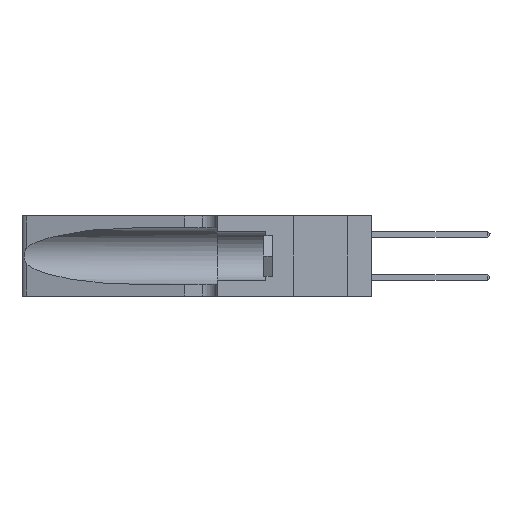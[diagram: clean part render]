
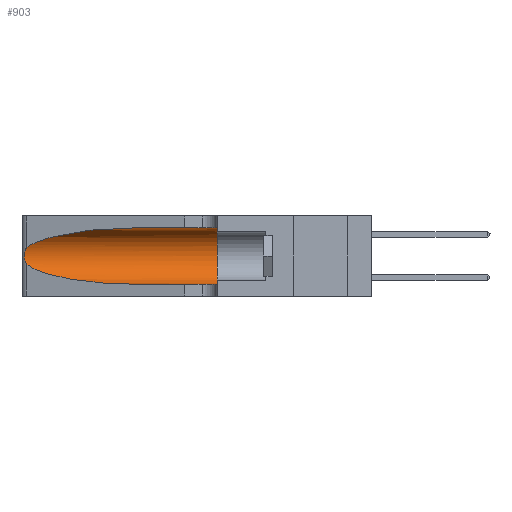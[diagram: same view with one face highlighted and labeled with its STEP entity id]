
A CAD part, left-side view. The second image highlights one B-rep face of the part: STEP entity #903.
In plain terms, the highlighted cylindrical face has radius 3.308 mm (diameter 6.617 mm), a partial arc.
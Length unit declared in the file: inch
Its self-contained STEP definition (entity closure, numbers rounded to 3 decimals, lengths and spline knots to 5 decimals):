
#76 = CARTESIAN_POINT ( 'NONE',  ( 0.1305, 0.72297, 0.05475 ) ) ;
#342 = DIRECTION ( 'NONE',  ( 0., 0., -1. ) ) ;
#652 = DIRECTION ( 'NONE',  ( 0., -1., 0. ) ) ;
#903 = ADVANCED_FACE ( 'NONE', ( #17242 ), #10014, .F. ) ;
#1303 = CARTESIAN_POINT ( 'NONE',  ( 0.25487, 1.22718, 0.22369 ) ) ;
#1406 = CARTESIAN_POINT ( 'NONE',  ( 0.26075, 1.23896, 0.19203 ) ) ;
#1470 = ORIENTED_EDGE ( 'NONE', *, *, #22122, .F. ) ;
#1732 = CARTESIAN_POINT ( 'NONE',  ( 0.1305, 0.72297, 0.31525 ) ) ;
#2048 = DIRECTION ( 'NONE',  ( 0., 1., 0. ) ) ;
#2212 = ORIENTED_EDGE ( 'NONE', *, *, #2371, .T. ) ;
#2371 = EDGE_CURVE ( 'NONE', #25575, #6496, #21791, .T. ) ;
#3704 = CARTESIAN_POINT ( 'NONE',  ( 0.26017, 1.23833, 0.17102 ) ) ;
#5071 = VECTOR ( 'NONE', #652, 39.37008 ) ;
#5984 = CARTESIAN_POINT ( 'NONE',  ( 0.25789, 1.23486, 0.15765 ) ) ;
#6429 = VERTEX_POINT ( 'NONE', #19236 ) ;
#6496 = VERTEX_POINT ( 'NONE', #10642 ) ;
#6513 = ORIENTED_EDGE ( 'NONE', *, *, #19465, .F. ) ;
#6844 = CARTESIAN_POINT ( 'NONE',  ( 0.18966, 0.96281, 0.05475 ) ) ;
#7109 = ORIENTED_EDGE ( 'NONE', *, *, #22461, .T. ) ;
#7920 = CARTESIAN_POINT ( 'NONE',  ( 0.2373, 1.15595, 0.28018 ) ) ;
#8261 = CARTESIAN_POINT ( 'NONE',  ( 0.25555, 1.22993, 0.14849 ) ) ;
#8276 = LINE ( 'NONE', #24031, #19307 ) ;
#9041 = EDGE_LOOP ( 'NONE', ( #11463, #26033, #2212, #7109, #6513, #1470 ) ) ;
#9395 = B_SPLINE_CURVE_WITH_KNOTS ( 'NONE', 3,
 ( #1303, #14700, #25813, #12568, #28002, #14795, #1406, #17002, #3704, #19243, #5984, #21479, #8261, #23672 ),
 .UNSPECIFIED., .F., .F.,
 ( 4, 2, 2, 2, 2, 2, 4 ),
 ( 0., 0.00027, 0.00053, 0.00107, 0.0016, 0.00187, 0.00214 ),
 .UNSPECIFIED. ) ;
#10014 = CYLINDRICAL_SURFACE ( 'NONE', #16537, 0.13025 ) ;
#10035 = CARTESIAN_POINT ( 'NONE',  ( 0.18966, 0.96281, 0.31525 ) ) ;
#10642 = CARTESIAN_POINT ( 'NONE',  ( 0.1305, 0.72297, 0.05475 ) ) ;
#11041 = CARTESIAN_POINT ( 'NONE',  ( 0.1305, 1.61858, 0.185 ) ) ;
#11463 = ORIENTED_EDGE ( 'NONE', *, *, #27934, .T. ) ;
#12116 = CARTESIAN_POINT ( 'NONE',  ( 0.25487, 1.22718, 0.22369 ) ) ;
#12568 = CARTESIAN_POINT ( 'NONE',  ( 0.25787, 1.23484, 0.2124 ) ) ;
#13022 = DIRECTION ( 'NONE',  ( 0., -1., 0. ) ) ;
#13495 = CARTESIAN_POINT ( 'NONE',  ( 0.25487, 1.22718, 0.14631 ) ) ;
#14700 = CARTESIAN_POINT ( 'NONE',  ( 0.25555, 1.22994, 0.2215 ) ) ;
#14795 = CARTESIAN_POINT ( 'NONE',  ( 0.26018, 1.23835, 0.19895 ) ) ;
#15414 = CARTESIAN_POINT ( 'NONE',  ( 0.1305, 0.35, 0.185 ) ) ;
#16537 = AXIS2_PLACEMENT_3D ( 'NONE', #11041, #18135, #342 ) ;
#16675 = CARTESIAN_POINT ( 'NONE',  ( 0.1305, 0.72297, 0.31525 ) ) ;
#17002 = CARTESIAN_POINT ( 'NONE',  ( 0.26075, 1.23896, 0.178 ) ) ;
#17242 = FACE_OUTER_BOUND ( 'NONE', #9041, .T. ) ;
#17512 =( BOUNDED_CURVE ( )  B_SPLINE_CURVE ( 3, ( #16675, #10035, #7920, #23343 ),
 .UNSPECIFIED., .F., .F. ) 
 B_SPLINE_CURVE_WITH_KNOTS ( ( 4, 4 ),
 ( 1.5708, 2.84003 ),
 .UNSPECIFIED. ) 
 CURVE ( )  GEOMETRIC_REPRESENTATION_ITEM ( )  RATIONAL_B_SPLINE_CURVE ( ( 1., 0.87, 0.87, 1. ) ) 
 REPRESENTATION_ITEM ( '' )  );
#17619 = DIRECTION ( 'NONE',  ( 0., 0., 1. ) ) ;
#18135 = DIRECTION ( 'NONE',  ( 0., -1., 0. ) ) ;
#19236 = CARTESIAN_POINT ( 'NONE',  ( 0.1305, 0.35, 0.05475 ) ) ;
#19243 = CARTESIAN_POINT ( 'NONE',  ( 0.25856, 1.23593, 0.16098 ) ) ;
#19307 = VECTOR ( 'NONE', #13022, 39.37008 ) ;
#19465 = EDGE_CURVE ( 'NONE', #21653, #6429, #25287, .T. ) ;
#20788 = AXIS2_PLACEMENT_3D ( 'NONE', #15414, #2048, #17619 ) ;
#21348 = EDGE_CURVE ( 'NONE', #25106, #25575, #9395, .T. ) ;
#21479 = CARTESIAN_POINT ( 'NONE',  ( 0.25639, 1.23186, 0.15144 ) ) ;
#21653 = VERTEX_POINT ( 'NONE', #26848 ) ;
#21791 =( BOUNDED_CURVE ( )  B_SPLINE_CURVE ( 3, ( #13495, #26737, #6844, #76 ),
 .UNSPECIFIED., .F., .T. ) 
 B_SPLINE_CURVE_WITH_KNOTS ( ( 4, 4 ),
 ( 3.44316, 4.71239 ),
 .UNSPECIFIED. ) 
 CURVE ( )  GEOMETRIC_REPRESENTATION_ITEM ( )  RATIONAL_B_SPLINE_CURVE ( ( 1., 0.87, 0.87, 1. ) ) 
 REPRESENTATION_ITEM ( '' )  );
#22122 = EDGE_CURVE ( 'NONE', #22760, #21653, #8276, .T. ) ;
#22461 = EDGE_CURVE ( 'NONE', #6496, #6429, #22737, .T. ) ;
#22529 = CARTESIAN_POINT ( 'NONE',  ( 0.25487, 1.22718, 0.14631 ) ) ;
#22737 = LINE ( 'NONE', #27289, #5071 ) ;
#22760 = VERTEX_POINT ( 'NONE', #1732 ) ;
#23343 = CARTESIAN_POINT ( 'NONE',  ( 0.25487, 1.22718, 0.22369 ) ) ;
#23672 = CARTESIAN_POINT ( 'NONE',  ( 0.25487, 1.22718, 0.14631 ) ) ;
#24031 = CARTESIAN_POINT ( 'NONE',  ( 0.1305, 1.61858, 0.31525 ) ) ;
#25106 = VERTEX_POINT ( 'NONE', #12116 ) ;
#25287 = CIRCLE ( 'NONE', #20788, 0.13025 ) ;
#25575 = VERTEX_POINT ( 'NONE', #22529 ) ;
#25813 = CARTESIAN_POINT ( 'NONE',  ( 0.25639, 1.23184, 0.21858 ) ) ;
#26033 = ORIENTED_EDGE ( 'NONE', *, *, #21348, .T. ) ;
#26737 = CARTESIAN_POINT ( 'NONE',  ( 0.2373, 1.15595, 0.08982 ) ) ;
#26848 = CARTESIAN_POINT ( 'NONE',  ( 0.1305, 0.35, 0.31525 ) ) ;
#27289 = CARTESIAN_POINT ( 'NONE',  ( 0.1305, 1.61858, 0.05475 ) ) ;
#27934 = EDGE_CURVE ( 'NONE', #22760, #25106, #17512, .T. ) ;
#28002 = CARTESIAN_POINT ( 'NONE',  ( 0.25854, 1.2359, 0.20912 ) ) ;
